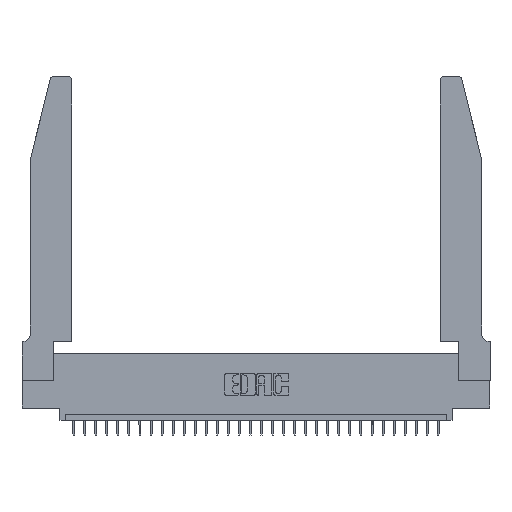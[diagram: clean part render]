
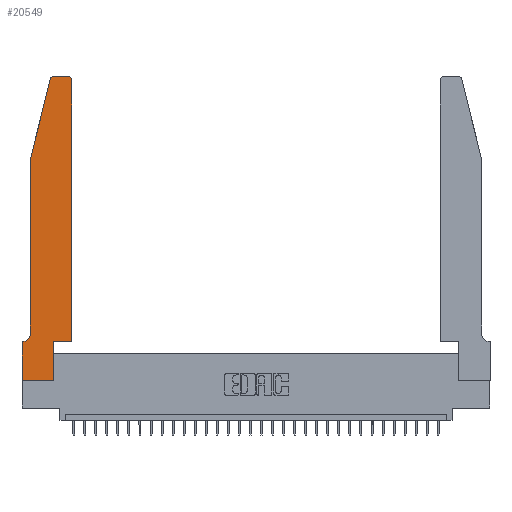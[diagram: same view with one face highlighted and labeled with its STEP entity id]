
A CAD part, top view. The second image highlights one B-rep face of the part: STEP entity #20549.
In plain terms, the highlighted planar face has unit normal (0, 0, 1).
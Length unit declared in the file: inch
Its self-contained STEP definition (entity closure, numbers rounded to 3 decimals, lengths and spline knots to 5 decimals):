
#94 = CARTESIAN_POINT ( 'NONE',  ( 0.4505, 2.72, 0.37 ) ) ;
#228 = CARTESIAN_POINT ( 'NONE',  ( 0.25487, 2.72718, 0.37 ) ) ;
#288 = CARTESIAN_POINT ( 'NONE',  ( 0.2865, 0.35, 0.37 ) ) ;
#297 = ORIENTED_EDGE ( 'NONE', *, *, #5203, .T. ) ;
#1822 = LINE ( 'NONE', #28245, #11847 ) ;
#2509 = EDGE_CURVE ( 'NONE', #6189, #28098, #26041, .T. ) ;
#2605 = CARTESIAN_POINT ( 'NONE',  ( 0.0755, 2., 0.37 ) ) ;
#2696 = CIRCLE ( 'NONE', #25176, 0.03 ) ;
#3120 = VERTEX_POINT ( 'NONE', #228 ) ;
#3124 = ORIENTED_EDGE ( 'NONE', *, *, #2509, .T. ) ;
#3647 = DIRECTION ( 'NONE',  ( -1., 0., 0. ) ) ;
#3748 = CARTESIAN_POINT ( 'NONE',  ( 0.2865, 0.35, 0.37 ) ) ;
#3960 = CARTESIAN_POINT ( 'NONE',  ( 0., 0., 0.37 ) ) ;
#4230 = ORIENTED_EDGE ( 'NONE', *, *, #22022, .T. ) ;
#4262 = DIRECTION ( 'NONE',  ( 0., -1., 0. ) ) ;
#4685 = EDGE_LOOP ( 'NONE', ( #30238, #297, #7270, #4230, #18786, #5992, #3124, #7268, #19957, #30641, #17549, #17691 ) ) ;
#5203 = EDGE_CURVE ( 'NONE', #10882, #3120, #2696, .T. ) ;
#5992 = ORIENTED_EDGE ( 'NONE', *, *, #13851, .T. ) ;
#6160 = DIRECTION ( 'NONE',  ( -1., 0., 0. ) ) ;
#6189 = VERTEX_POINT ( 'NONE', #7060 ) ;
#6210 = CARTESIAN_POINT ( 'NONE',  ( 0.0055, 0.35, 0.37 ) ) ;
#6314 = PLANE ( 'NONE',  #14406 ) ;
#6469 = DIRECTION ( 'NONE',  ( 0., 0., 1. ) ) ;
#6617 = LINE ( 'NONE', #10956, #7795 ) ;
#6766 = DIRECTION ( 'NONE',  ( 0., 1., 0. ) ) ;
#7060 = CARTESIAN_POINT ( 'NONE',  ( 0., 0.35, 0.37 ) ) ;
#7268 = ORIENTED_EDGE ( 'NONE', *, *, #13196, .T. ) ;
#7270 = ORIENTED_EDGE ( 'NONE', *, *, #10379, .T. ) ;
#7510 = CIRCLE ( 'NONE', #18250, 0.07 ) ;
#7795 = VECTOR ( 'NONE', #6766, 39.37008 ) ;
#8778 = EDGE_CURVE ( 'NONE', #17220, #24110, #18298, .T. ) ;
#9087 = CARTESIAN_POINT ( 'NONE',  ( 0.2865, 0., 0.37 ) ) ;
#9444 = LINE ( 'NONE', #2605, #31576 ) ;
#9456 = CARTESIAN_POINT ( 'NONE',  ( 0.4505, 0.35, 0.37 ) ) ;
#9940 = DIRECTION ( 'NONE',  ( -0.239, -0.971, 0. ) ) ;
#10129 = CARTESIAN_POINT ( 'NONE',  ( 0.4205, 2.75, 0.37 ) ) ;
#10271 = CARTESIAN_POINT ( 'NONE',  ( 0., 0., 0.37 ) ) ;
#10379 = EDGE_CURVE ( 'NONE', #3120, #31349, #9444, .T. ) ;
#10882 = VERTEX_POINT ( 'NONE', #17611 ) ;
#10956 = CARTESIAN_POINT ( 'NONE',  ( 0.4505, 0.35, 0.37 ) ) ;
#11145 = CARTESIAN_POINT ( 'NONE',  ( 0.0755, 2., 0.37 ) ) ;
#11563 = VECTOR ( 'NONE', #22143, 39.37008 ) ;
#11847 = VECTOR ( 'NONE', #6160, 39.37008 ) ;
#12114 = LINE ( 'NONE', #21575, #24859 ) ;
#12144 = VERTEX_POINT ( 'NONE', #6210 ) ;
#12284 = DIRECTION ( 'NONE',  ( 0., -1., 0. ) ) ;
#13196 = EDGE_CURVE ( 'NONE', #28098, #31142, #22610, .T. ) ;
#13490 = DIRECTION ( 'NONE',  ( 0., 1., 0. ) ) ;
#13851 = EDGE_CURVE ( 'NONE', #12144, #6189, #1822, .T. ) ;
#13863 = EDGE_CURVE ( 'NONE', #21994, #17220, #6617, .T. ) ;
#14406 = AXIS2_PLACEMENT_3D ( 'NONE', #28864, #14963, #26800 ) ;
#14514 = LINE ( 'NONE', #31494, #19116 ) ;
#14751 = DIRECTION ( 'NONE',  ( 1., 0., 0. ) ) ;
#14963 = DIRECTION ( 'NONE',  ( 0., 0., 1. ) ) ;
#15477 = EDGE_CURVE ( 'NONE', #31142, #28239, #18306, .T. ) ;
#16539 = DIRECTION ( 'NONE',  ( 1., 0., 0. ) ) ;
#17220 = VERTEX_POINT ( 'NONE', #94 ) ;
#17549 = ORIENTED_EDGE ( 'NONE', *, *, #13863, .T. ) ;
#17611 = CARTESIAN_POINT ( 'NONE',  ( 0.284, 2.75, 0.37 ) ) ;
#17691 = ORIENTED_EDGE ( 'NONE', *, *, #8778, .T. ) ;
#18196 = DIRECTION ( 'NONE',  ( 0., 0., -1. ) ) ;
#18250 = AXIS2_PLACEMENT_3D ( 'NONE', #30531, #18196, #3647 ) ;
#18298 = CIRCLE ( 'NONE', #22415, 0.03 ) ;
#18306 = LINE ( 'NONE', #3748, #26035 ) ;
#18498 = FACE_OUTER_BOUND ( 'NONE', #4685, .T. ) ;
#18512 = CARTESIAN_POINT ( 'NONE',  ( 0.0755, 0.42, 0.37 ) ) ;
#18786 = ORIENTED_EDGE ( 'NONE', *, *, #29448, .T. ) ;
#19116 = VECTOR ( 'NONE', #12284, 39.37008 ) ;
#19254 = VECTOR ( 'NONE', #4262, 39.37008 ) ;
#19332 = CARTESIAN_POINT ( 'NONE',  ( 0.4505, 0.35, 0.37 ) ) ;
#19957 = ORIENTED_EDGE ( 'NONE', *, *, #15477, .T. ) ;
#20549 = ADVANCED_FACE ( 'NONE', ( #18498 ), #6314, .T. ) ;
#21080 = CARTESIAN_POINT ( 'NONE',  ( 0.4205, 2.72, 0.37 ) ) ;
#21112 = CARTESIAN_POINT ( 'NONE',  ( 0., 0., 0.37 ) ) ;
#21575 = CARTESIAN_POINT ( 'NONE',  ( 0.2605, 2.75, 0.37 ) ) ;
#21682 = CARTESIAN_POINT ( 'NONE',  ( 0.284, 2.72, 0.37 ) ) ;
#21896 = DIRECTION ( 'NONE',  ( -1., 0., 0. ) ) ;
#21994 = VERTEX_POINT ( 'NONE', #19332 ) ;
#22022 = EDGE_CURVE ( 'NONE', #31349, #22351, #14514, .T. ) ;
#22143 = DIRECTION ( 'NONE',  ( 1., 0., 0. ) ) ;
#22351 = VERTEX_POINT ( 'NONE', #18512 ) ;
#22415 = AXIS2_PLACEMENT_3D ( 'NONE', #21080, #23929, #26030 ) ;
#22610 = LINE ( 'NONE', #10271, #31264 ) ;
#23929 = DIRECTION ( 'NONE',  ( 0., 0., 1. ) ) ;
#24110 = VERTEX_POINT ( 'NONE', #10129 ) ;
#24543 = LINE ( 'NONE', #9456, #11563 ) ;
#24859 = VECTOR ( 'NONE', #21896, 39.37008 ) ;
#25176 = AXIS2_PLACEMENT_3D ( 'NONE', #21682, #6469, #16539 ) ;
#25231 = EDGE_CURVE ( 'NONE', #28239, #21994, #24543, .T. ) ;
#26030 = DIRECTION ( 'NONE',  ( 1., 0., 0. ) ) ;
#26035 = VECTOR ( 'NONE', #13490, 39.37008 ) ;
#26041 = LINE ( 'NONE', #3960, #19254 ) ;
#26800 = DIRECTION ( 'NONE',  ( 1., 0., 0. ) ) ;
#28098 = VERTEX_POINT ( 'NONE', #21112 ) ;
#28189 = EDGE_CURVE ( 'NONE', #24110, #10882, #12114, .T. ) ;
#28239 = VERTEX_POINT ( 'NONE', #288 ) ;
#28245 = CARTESIAN_POINT ( 'NONE',  ( 0.0755, 0.35, 0.37 ) ) ;
#28864 = CARTESIAN_POINT ( 'NONE',  ( 0., 0.35, 0.37 ) ) ;
#29448 = EDGE_CURVE ( 'NONE', #22351, #12144, #7510, .T. ) ;
#30238 = ORIENTED_EDGE ( 'NONE', *, *, #28189, .T. ) ;
#30531 = CARTESIAN_POINT ( 'NONE',  ( 0.0055, 0.42, 0.37 ) ) ;
#30641 = ORIENTED_EDGE ( 'NONE', *, *, #25231, .T. ) ;
#31142 = VERTEX_POINT ( 'NONE', #9087 ) ;
#31264 = VECTOR ( 'NONE', #14751, 39.37008 ) ;
#31349 = VERTEX_POINT ( 'NONE', #11145 ) ;
#31494 = CARTESIAN_POINT ( 'NONE',  ( 0.0755, 2., 0.37 ) ) ;
#31576 = VECTOR ( 'NONE', #9940, 39.37008 ) ;
